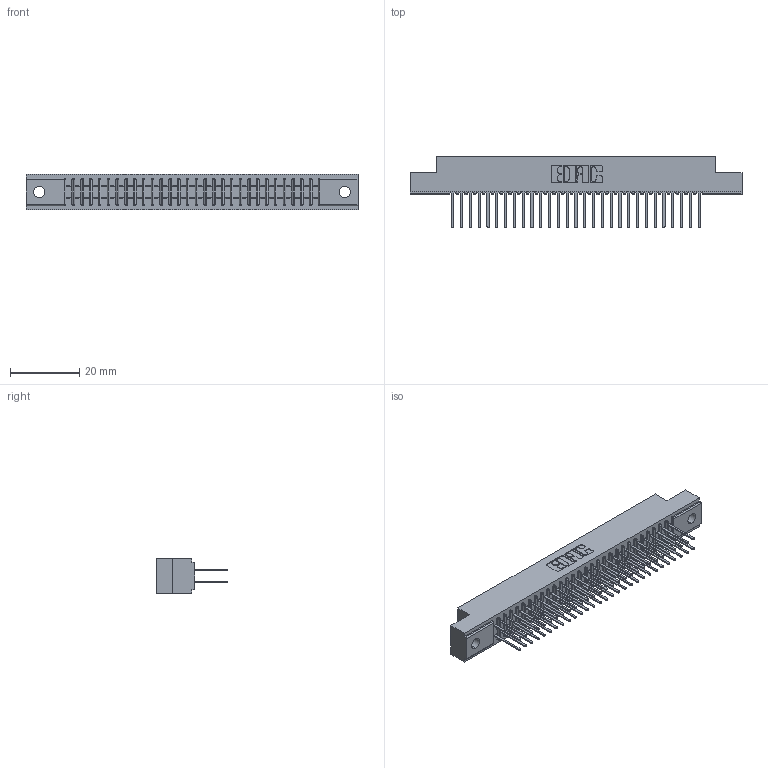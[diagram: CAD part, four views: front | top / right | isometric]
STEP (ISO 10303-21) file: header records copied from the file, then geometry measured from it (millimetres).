
FILE_DESCRIPTION (( 'STEP AP203' ), '1' );
FILE_NAME ('341-058-522-202.STEP', '2018-08-07T16:20:40', ( '' ), ( '' ), 'SwSTEP 2.0', 'SolidWorks 2016', '' );
FILE_SCHEMA (( 'CONFIG_CONTROL_DESIGN' ));
Length unit declared in the file: inch
Products named in the file (3): 341 Part_.128 (3.25) Dia Mounting Holes; 341-292-001_341-292-122; 341-058-522-202
Assembly tree (59 placements, depth 2):
  341-058-522-202
    341 Part_.128 (3.25) Dia Mounting Holes
    341-292-001_341-292-122  x58
Bounding box: 95.89 x 20.62 x 10.16 mm (x, y, z)
Volume: 7108.5 mm3; surface area: 12476.7 mm2
Topology: 59 solids, 59 shells, 3944 faces, 11423 edges, 7398 vertices
Faces by surface type: plane 2388, cylinder 1440, sphere 60, torus 56
Entity records: 36830 total; most frequent: CARTESIAN_POINT 6123, ORIENTED_EDGE 6082, DIRECTION 5951, EDGE_CURVE 3041, VECTOR 2443, LINE 2443, VERTEX_POINT 1926, AXIS2_PLACEMENT_3D 1754
